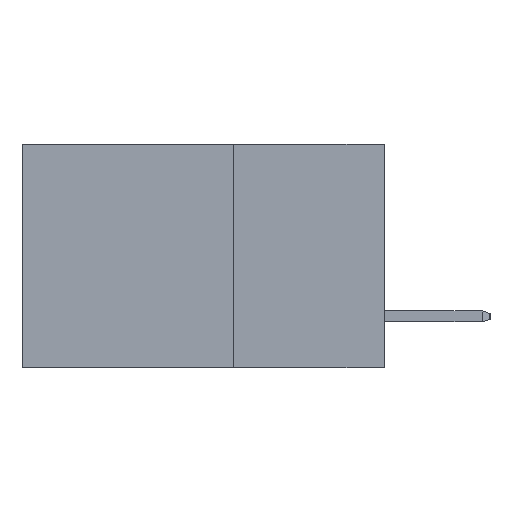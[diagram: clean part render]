
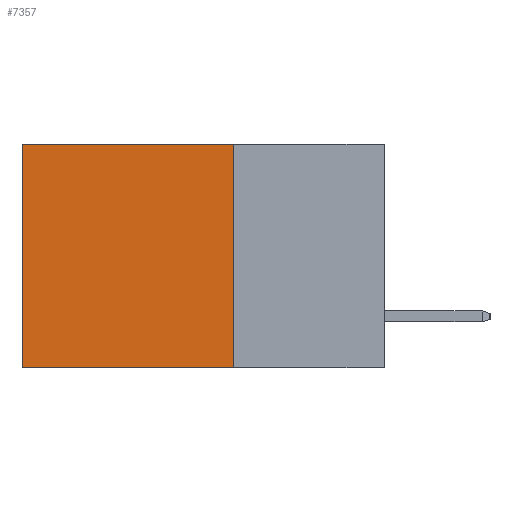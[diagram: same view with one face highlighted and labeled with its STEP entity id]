
A CAD part, left-side view. The second image highlights one B-rep face of the part: STEP entity #7357.
In plain terms, the highlighted planar face has unit normal (-1, 0, 0).
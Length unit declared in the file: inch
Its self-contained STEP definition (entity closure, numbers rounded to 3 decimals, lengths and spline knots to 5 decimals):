
#195 = LINE ( 'NONE', #8243, #14023 ) ;
#392 = CARTESIAN_POINT ( 'NONE',  ( 0.2615, 0.25, 0. ) ) ;
#1252 = DIRECTION ( 'NONE',  ( 0., 0., -1. ) ) ;
#1420 = VERTEX_POINT ( 'NONE', #13160 ) ;
#2552 = EDGE_CURVE ( 'NONE', #2706, #17395, #17195, .T. ) ;
#2706 = VERTEX_POINT ( 'NONE', #20657 ) ;
#2804 = CARTESIAN_POINT ( 'NONE',  ( 0.2615, 0.6, -0.37 ) ) ;
#3516 = EDGE_CURVE ( 'NONE', #1420, #17395, #14924, .T. ) ;
#4029 = FACE_OUTER_BOUND ( 'NONE', #11488, .T. ) ;
#5435 = VECTOR ( 'NONE', #9889, 39.37008 ) ;
#5507 = VECTOR ( 'NONE', #12521, 39.37008 ) ;
#6175 = ORIENTED_EDGE ( 'NONE', *, *, #10312, .T. ) ;
#6728 = ORIENTED_EDGE ( 'NONE', *, *, #2552, .T. ) ;
#7357 = ADVANCED_FACE ( 'NONE', ( #4029 ), #15142, .F. ) ;
#8162 = DIRECTION ( 'NONE',  ( 0., 0., -1. ) ) ;
#8243 = CARTESIAN_POINT ( 'NONE',  ( 0.2615, 0.25, -0.37 ) ) ;
#8454 = AXIS2_PLACEMENT_3D ( 'NONE', #13868, #14989, #15409 ) ;
#9620 = CARTESIAN_POINT ( 'NONE',  ( 0.2615, 0.25, -0.37 ) ) ;
#9889 = DIRECTION ( 'NONE',  ( 0., 1., 0. ) ) ;
#10249 = LINE ( 'NONE', #12863, #5507 ) ;
#10312 = EDGE_CURVE ( 'NONE', #13324, #2706, #10249, .T. ) ;
#11488 = EDGE_LOOP ( 'NONE', ( #6728, #18879, #14781, #6175 ) ) ;
#11905 = VECTOR ( 'NONE', #1252, 39.37008 ) ;
#12521 = DIRECTION ( 'NONE',  ( 0., 1., 0. ) ) ;
#12705 = EDGE_CURVE ( 'NONE', #13324, #1420, #195, .T. ) ;
#12863 = CARTESIAN_POINT ( 'NONE',  ( 0.2615, 0.25, 0. ) ) ;
#13160 = CARTESIAN_POINT ( 'NONE',  ( 0.2615, 0.25, -0.37 ) ) ;
#13324 = VERTEX_POINT ( 'NONE', #392 ) ;
#13868 = CARTESIAN_POINT ( 'NONE',  ( 0.2615, 0.25, -0.37 ) ) ;
#14023 = VECTOR ( 'NONE', #8162, 39.37008 ) ;
#14781 = ORIENTED_EDGE ( 'NONE', *, *, #12705, .F. ) ;
#14924 = LINE ( 'NONE', #9620, #5435 ) ;
#14989 = DIRECTION ( 'NONE',  ( 1., 0., 0. ) ) ;
#15142 = PLANE ( 'NONE',  #8454 ) ;
#15409 = DIRECTION ( 'NONE',  ( 0., 0., -1. ) ) ;
#17195 = LINE ( 'NONE', #22922, #11905 ) ;
#17395 = VERTEX_POINT ( 'NONE', #2804 ) ;
#18879 = ORIENTED_EDGE ( 'NONE', *, *, #3516, .F. ) ;
#20657 = CARTESIAN_POINT ( 'NONE',  ( 0.2615, 0.6, 0. ) ) ;
#22922 = CARTESIAN_POINT ( 'NONE',  ( 0.2615, 0.6, -0.37 ) ) ;
